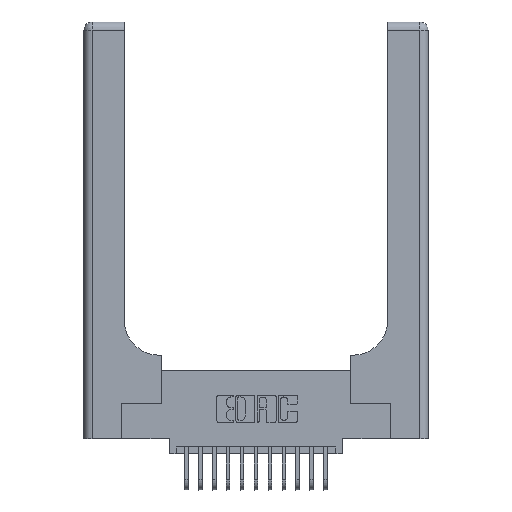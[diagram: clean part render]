
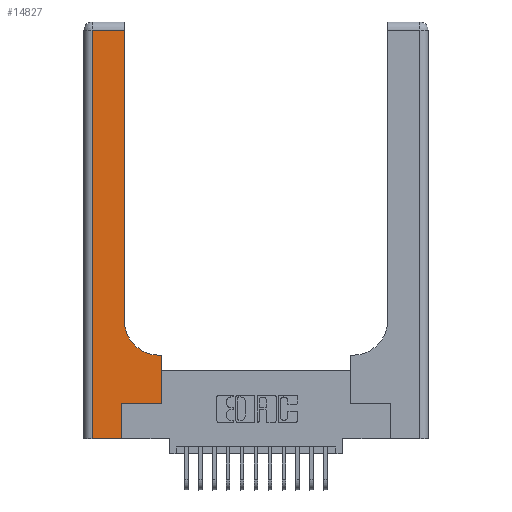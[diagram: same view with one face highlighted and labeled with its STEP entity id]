
A CAD part, top view. The second image highlights one B-rep face of the part: STEP entity #14827.
In plain terms, the highlighted planar face has unit normal (0, 0, 1).
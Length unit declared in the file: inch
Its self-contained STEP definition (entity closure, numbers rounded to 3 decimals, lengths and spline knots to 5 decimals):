
#137 = CIRCLE ( 'NONE', #7406, 0.25 ) ;
#164 = DIRECTION ( 'NONE',  ( 0., 0., -1. ) ) ;
#359 = ORIENTED_EDGE ( 'NONE', *, *, #11120, .T. ) ;
#1062 = DIRECTION ( 'NONE',  ( 1., 0., 0. ) ) ;
#1072 = VECTOR ( 'NONE', #18423, 39.37008 ) ;
#2020 = VECTOR ( 'NONE', #1062, 39.37008 ) ;
#2234 = LINE ( 'NONE', #11521, #13702 ) ;
#2988 = DIRECTION ( 'NONE',  ( 0., 1., 0. ) ) ;
#3051 = ORIENTED_EDGE ( 'NONE', *, *, #5272, .T. ) ;
#3678 = VERTEX_POINT ( 'NONE', #19171 ) ;
#4074 = CARTESIAN_POINT ( 'NONE',  ( 0.269, 0., 0.37 ) ) ;
#4169 = CARTESIAN_POINT ( 'NONE',  ( 0., 0., 0.37 ) ) ;
#4293 = VECTOR ( 'NONE', #2988, 39.37008 ) ;
#4471 = CARTESIAN_POINT ( 'NONE',  ( 0.5585, 0.6, 0.37 ) ) ;
#4556 = CARTESIAN_POINT ( 'NONE',  ( 0.2915, 0.6, 0.37 ) ) ;
#4643 = LINE ( 'NONE', #6384, #11142 ) ;
#5208 = CARTESIAN_POINT ( 'NONE',  ( 0.5415, 0.85, 0.37 ) ) ;
#5272 = EDGE_CURVE ( 'NONE', #3678, #15783, #4643, .T. ) ;
#5482 = VERTEX_POINT ( 'NONE', #4471 ) ;
#6054 = CARTESIAN_POINT ( 'NONE',  ( 0.5585, 0.25, 0.37 ) ) ;
#6072 = EDGE_CURVE ( 'NONE', #15089, #18798, #14926, .T. ) ;
#6242 = VERTEX_POINT ( 'NONE', #18675 ) ;
#6352 = EDGE_CURVE ( 'NONE', #6242, #15089, #2234, .T. ) ;
#6384 = CARTESIAN_POINT ( 'NONE',  ( 0.269, 0.25, 0.37 ) ) ;
#6954 = EDGE_CURVE ( 'NONE', #7601, #6242, #12747, .T. ) ;
#7199 = ORIENTED_EDGE ( 'NONE', *, *, #11355, .T. ) ;
#7406 = AXIS2_PLACEMENT_3D ( 'NONE', #5208, #8323, #19000 ) ;
#7510 = VERTEX_POINT ( 'NONE', #16665 ) ;
#7600 = ORIENTED_EDGE ( 'NONE', *, *, #6954, .T. ) ;
#7601 = VERTEX_POINT ( 'NONE', #16547 ) ;
#7793 = CARTESIAN_POINT ( 'NONE',  ( 0., 3., 0.37 ) ) ;
#8069 = ORIENTED_EDGE ( 'NONE', *, *, #6072, .T. ) ;
#8247 = LINE ( 'NONE', #14003, #15915 ) ;
#8323 = DIRECTION ( 'NONE',  ( 0., 0., -1. ) ) ;
#8327 = ORIENTED_EDGE ( 'NONE', *, *, #8622, .T. ) ;
#8622 = EDGE_CURVE ( 'NONE', #18798, #3678, #13874, .T. ) ;
#9025 = CARTESIAN_POINT ( 'NONE',  ( 0.5585, 0.25, 0.37 ) ) ;
#9427 = LINE ( 'NONE', #4556, #1072 ) ;
#9795 = DIRECTION ( 'NONE',  ( 0., -1., 0. ) ) ;
#9819 = VECTOR ( 'NONE', #12349, 39.37008 ) ;
#9848 = LINE ( 'NONE', #6054, #4293 ) ;
#10340 = DIRECTION ( 'NONE',  ( -1., 0., 0. ) ) ;
#10575 = CARTESIAN_POINT ( 'NONE',  ( 0.5415, 0.6, 0.37 ) ) ;
#10648 = EDGE_LOOP ( 'NONE', ( #359, #7600, #15883, #8069, #8327, #3051, #19498, #16384, #7199 ) ) ;
#11120 = EDGE_CURVE ( 'NONE', #7510, #7601, #8247, .T. ) ;
#11142 = VECTOR ( 'NONE', #18281, 39.37008 ) ;
#11355 = EDGE_CURVE ( 'NONE', #16206, #7510, #137, .T. ) ;
#11521 = CARTESIAN_POINT ( 'NONE',  ( 0.06, 3., 0.37 ) ) ;
#11831 = EDGE_CURVE ( 'NONE', #5482, #16206, #9427, .T. ) ;
#12327 = DIRECTION ( 'NONE',  ( -1., 0., 0. ) ) ;
#12349 = DIRECTION ( 'NONE',  ( 0., 1., 0. ) ) ;
#12465 = PLANE ( 'NONE',  #19214 ) ;
#12747 = LINE ( 'NONE', #14878, #18461 ) ;
#13702 = VECTOR ( 'NONE', #9795, 39.37008 ) ;
#13866 = FACE_OUTER_BOUND ( 'NONE', #10648, .T. ) ;
#13874 = LINE ( 'NONE', #13940, #9819 ) ;
#13940 = CARTESIAN_POINT ( 'NONE',  ( 0.269, 0., 0.37 ) ) ;
#13946 = EDGE_CURVE ( 'NONE', #15783, #5482, #9848, .T. ) ;
#14003 = CARTESIAN_POINT ( 'NONE',  ( 0.2915, 3., 0.37 ) ) ;
#14827 = ADVANCED_FACE ( 'NONE', ( #13866 ), #12465, .F. ) ;
#14878 = CARTESIAN_POINT ( 'NONE',  ( 0., 2.94, 0.37 ) ) ;
#14926 = LINE ( 'NONE', #4169, #2020 ) ;
#15089 = VERTEX_POINT ( 'NONE', #19177 ) ;
#15783 = VERTEX_POINT ( 'NONE', #9025 ) ;
#15883 = ORIENTED_EDGE ( 'NONE', *, *, #6352, .T. ) ;
#15915 = VECTOR ( 'NONE', #17060, 39.37008 ) ;
#16206 = VERTEX_POINT ( 'NONE', #10575 ) ;
#16384 = ORIENTED_EDGE ( 'NONE', *, *, #11831, .T. ) ;
#16547 = CARTESIAN_POINT ( 'NONE',  ( 0.2915, 2.94, 0.37 ) ) ;
#16665 = CARTESIAN_POINT ( 'NONE',  ( 0.2915, 0.85, 0.37 ) ) ;
#17060 = DIRECTION ( 'NONE',  ( 0., 1., 0. ) ) ;
#18281 = DIRECTION ( 'NONE',  ( 1., 0., 0. ) ) ;
#18423 = DIRECTION ( 'NONE',  ( -1., 0., 0. ) ) ;
#18461 = VECTOR ( 'NONE', #10340, 39.37008 ) ;
#18675 = CARTESIAN_POINT ( 'NONE',  ( 0.06, 2.94, 0.37 ) ) ;
#18798 = VERTEX_POINT ( 'NONE', #4074 ) ;
#19000 = DIRECTION ( 'NONE',  ( 1., 0., 0. ) ) ;
#19171 = CARTESIAN_POINT ( 'NONE',  ( 0.269, 0.25, 0.37 ) ) ;
#19177 = CARTESIAN_POINT ( 'NONE',  ( 0.06, 0., 0.37 ) ) ;
#19214 = AXIS2_PLACEMENT_3D ( 'NONE', #7793, #164, #12327 ) ;
#19498 = ORIENTED_EDGE ( 'NONE', *, *, #13946, .T. ) ;
